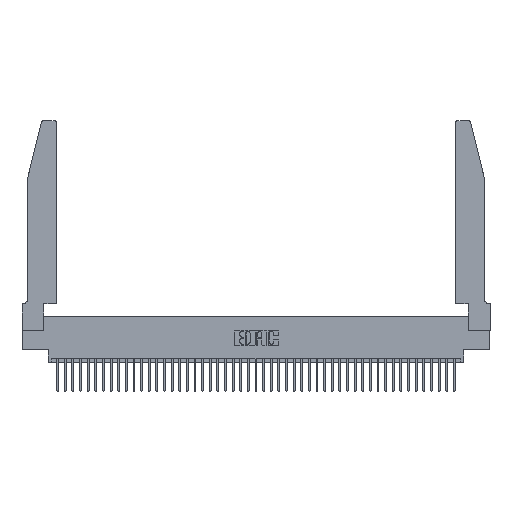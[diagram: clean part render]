
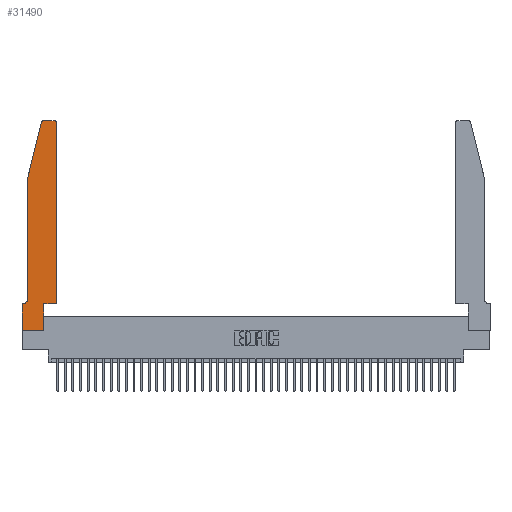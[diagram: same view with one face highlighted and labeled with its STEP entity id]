
A CAD part, top view. The second image highlights one B-rep face of the part: STEP entity #31490.
In plain terms, the highlighted planar face has unit normal (0, 0, 1).
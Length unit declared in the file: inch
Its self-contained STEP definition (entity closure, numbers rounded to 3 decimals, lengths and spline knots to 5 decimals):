
#122 = ORIENTED_EDGE ( 'NONE', *, *, #14981, .T. ) ;
#131 = AXIS2_PLACEMENT_3D ( 'NONE', #32396, #32083, #39551 ) ;
#266 = CARTESIAN_POINT ( 'NONE',  ( 0., 0., 0.37 ) ) ;
#344 = VERTEX_POINT ( 'NONE', #266 ) ;
#371 = VECTOR ( 'NONE', #37389, 39.37008 ) ;
#493 = LINE ( 'NONE', #6004, #3268 ) ;
#662 = CARTESIAN_POINT ( 'NONE',  ( 0.0755, 2., 0.37 ) ) ;
#692 = DIRECTION ( 'NONE',  ( 0., 1., 0. ) ) ;
#2466 = LINE ( 'NONE', #31133, #13912 ) ;
#3268 = VECTOR ( 'NONE', #34278, 39.37008 ) ;
#3992 = CARTESIAN_POINT ( 'NONE',  ( 0., 0.35, 0.37 ) ) ;
#4207 = VERTEX_POINT ( 'NONE', #3992 ) ;
#4444 = DIRECTION ( 'NONE',  ( 0., 0., 1. ) ) ;
#4799 = VERTEX_POINT ( 'NONE', #12134 ) ;
#5060 = CARTESIAN_POINT ( 'NONE',  ( 0.0755, 0.42, 0.37 ) ) ;
#5951 = CIRCLE ( 'NONE', #22077, 0.03 ) ;
#6004 = CARTESIAN_POINT ( 'NONE',  ( 0., 0., 0.37 ) ) ;
#6734 = DIRECTION ( 'NONE',  ( 0., -1., 0. ) ) ;
#6756 = CIRCLE ( 'NONE', #19233, 0.03 ) ;
#7800 = LINE ( 'NONE', #662, #24718 ) ;
#7810 = VERTEX_POINT ( 'NONE', #43664 ) ;
#9565 = CARTESIAN_POINT ( 'NONE',  ( 0.4205, 2.75, 0.37 ) ) ;
#10540 = ORIENTED_EDGE ( 'NONE', *, *, #13833, .T. ) ;
#11594 = CARTESIAN_POINT ( 'NONE',  ( 0., 0.35, 0.37 ) ) ;
#11911 = DIRECTION ( 'NONE',  ( 0., 1., 0. ) ) ;
#12134 = CARTESIAN_POINT ( 'NONE',  ( 0.0755, 2., 0.37 ) ) ;
#12741 = CARTESIAN_POINT ( 'NONE',  ( 0.284, 2.75, 0.37 ) ) ;
#12882 = DIRECTION ( 'NONE',  ( 1., 0., 0. ) ) ;
#13506 = LINE ( 'NONE', #35958, #35232 ) ;
#13753 = VERTEX_POINT ( 'NONE', #9565 ) ;
#13833 = EDGE_CURVE ( 'NONE', #28907, #7810, #15775, .T. ) ;
#13912 = VECTOR ( 'NONE', #44852, 39.37008 ) ;
#14045 = LINE ( 'NONE', #44385, #371 ) ;
#14304 = ORIENTED_EDGE ( 'NONE', *, *, #29888, .T. ) ;
#14630 = LINE ( 'NONE', #18368, #17883 ) ;
#14981 = EDGE_CURVE ( 'NONE', #4799, #15901, #13506, .T. ) ;
#15612 = EDGE_CURVE ( 'NONE', #15901, #42066, #16710, .T. ) ;
#15775 = LINE ( 'NONE', #36485, #27194 ) ;
#15901 = VERTEX_POINT ( 'NONE', #5060 ) ;
#16453 = ORIENTED_EDGE ( 'NONE', *, *, #36016, .T. ) ;
#16710 = CIRCLE ( 'NONE', #131, 0.07 ) ;
#16727 = VERTEX_POINT ( 'NONE', #12741 ) ;
#16975 = ORIENTED_EDGE ( 'NONE', *, *, #31848, .T. ) ;
#17883 = VECTOR ( 'NONE', #692, 39.37008 ) ;
#17894 = EDGE_LOOP ( 'NONE', ( #29249, #32715, #14304, #122, #44858, #43128, #21734, #16975, #24215, #10540, #25795, #16453 ) ) ;
#17975 = CARTESIAN_POINT ( 'NONE',  ( 0.4205, 2.72, 0.37 ) ) ;
#18368 = CARTESIAN_POINT ( 'NONE',  ( 0.2865, 0.35, 0.37 ) ) ;
#19233 = AXIS2_PLACEMENT_3D ( 'NONE', #17975, #42300, #38391 ) ;
#20474 = DIRECTION ( 'NONE',  ( -1., 0., 0. ) ) ;
#21734 = ORIENTED_EDGE ( 'NONE', *, *, #44191, .T. ) ;
#22077 = AXIS2_PLACEMENT_3D ( 'NONE', #43915, #23515, #12882 ) ;
#23265 = AXIS2_PLACEMENT_3D ( 'NONE', #11594, #4444, #28925 ) ;
#23515 = DIRECTION ( 'NONE',  ( 0., 0., 1. ) ) ;
#24188 = CARTESIAN_POINT ( 'NONE',  ( 0.2865, 0., 0.37 ) ) ;
#24215 = ORIENTED_EDGE ( 'NONE', *, *, #32094, .T. ) ;
#24718 = VECTOR ( 'NONE', #35835, 39.37008 ) ;
#25270 = PLANE ( 'NONE',  #23265 ) ;
#25594 = CARTESIAN_POINT ( 'NONE',  ( 0.4505, 0.35, 0.37 ) ) ;
#25795 = ORIENTED_EDGE ( 'NONE', *, *, #27388, .T. ) ;
#27194 = VECTOR ( 'NONE', #43634, 39.37008 ) ;
#27388 = EDGE_CURVE ( 'NONE', #7810, #41963, #29843, .T. ) ;
#27742 = VERTEX_POINT ( 'NONE', #24188 ) ;
#28102 = LINE ( 'NONE', #31256, #32437 ) ;
#28373 = FACE_OUTER_BOUND ( 'NONE', #17894, .T. ) ;
#28907 = VERTEX_POINT ( 'NONE', #37409 ) ;
#28925 = DIRECTION ( 'NONE',  ( 1., 0., 0. ) ) ;
#29245 = CARTESIAN_POINT ( 'NONE',  ( 0.25487, 2.72718, 0.37 ) ) ;
#29249 = ORIENTED_EDGE ( 'NONE', *, *, #30085, .T. ) ;
#29380 = CARTESIAN_POINT ( 'NONE',  ( 0.4505, 2.72, 0.37 ) ) ;
#29843 = LINE ( 'NONE', #25594, #41271 ) ;
#29888 = EDGE_CURVE ( 'NONE', #33630, #4799, #7800, .T. ) ;
#30085 = EDGE_CURVE ( 'NONE', #13753, #16727, #2466, .T. ) ;
#31133 = CARTESIAN_POINT ( 'NONE',  ( 0.2605, 2.75, 0.37 ) ) ;
#31256 = CARTESIAN_POINT ( 'NONE',  ( 0.0755, 0.35, 0.37 ) ) ;
#31490 = ADVANCED_FACE ( 'NONE', ( #28373 ), #25270, .T. ) ;
#31848 = EDGE_CURVE ( 'NONE', #344, #27742, #493, .T. ) ;
#32083 = DIRECTION ( 'NONE',  ( 0., 0., -1. ) ) ;
#32094 = EDGE_CURVE ( 'NONE', #27742, #28907, #14630, .T. ) ;
#32396 = CARTESIAN_POINT ( 'NONE',  ( 0.0055, 0.42, 0.37 ) ) ;
#32437 = VECTOR ( 'NONE', #20474, 39.37008 ) ;
#32715 = ORIENTED_EDGE ( 'NONE', *, *, #33256, .T. ) ;
#33256 = EDGE_CURVE ( 'NONE', #16727, #33630, #5951, .T. ) ;
#33630 = VERTEX_POINT ( 'NONE', #29245 ) ;
#33678 = CARTESIAN_POINT ( 'NONE',  ( 0.0055, 0.35, 0.37 ) ) ;
#34278 = DIRECTION ( 'NONE',  ( 1., 0., 0. ) ) ;
#35232 = VECTOR ( 'NONE', #6734, 39.37008 ) ;
#35835 = DIRECTION ( 'NONE',  ( -0.239, -0.971, 0. ) ) ;
#35958 = CARTESIAN_POINT ( 'NONE',  ( 0.0755, 2., 0.37 ) ) ;
#36016 = EDGE_CURVE ( 'NONE', #41963, #13753, #6756, .T. ) ;
#36485 = CARTESIAN_POINT ( 'NONE',  ( 0.4505, 0.35, 0.37 ) ) ;
#37389 = DIRECTION ( 'NONE',  ( 0., -1., 0. ) ) ;
#37409 = CARTESIAN_POINT ( 'NONE',  ( 0.2865, 0.35, 0.37 ) ) ;
#38391 = DIRECTION ( 'NONE',  ( 1., 0., 0. ) ) ;
#39551 = DIRECTION ( 'NONE',  ( -1., 0., 0. ) ) ;
#41271 = VECTOR ( 'NONE', #11911, 39.37008 ) ;
#41963 = VERTEX_POINT ( 'NONE', #29380 ) ;
#42066 = VERTEX_POINT ( 'NONE', #33678 ) ;
#42300 = DIRECTION ( 'NONE',  ( 0., 0., 1. ) ) ;
#43128 = ORIENTED_EDGE ( 'NONE', *, *, #44364, .T. ) ;
#43634 = DIRECTION ( 'NONE',  ( 1., 0., 0. ) ) ;
#43664 = CARTESIAN_POINT ( 'NONE',  ( 0.4505, 0.35, 0.37 ) ) ;
#43915 = CARTESIAN_POINT ( 'NONE',  ( 0.284, 2.72, 0.37 ) ) ;
#44191 = EDGE_CURVE ( 'NONE', #4207, #344, #14045, .T. ) ;
#44364 = EDGE_CURVE ( 'NONE', #42066, #4207, #28102, .T. ) ;
#44385 = CARTESIAN_POINT ( 'NONE',  ( 0., 0., 0.37 ) ) ;
#44852 = DIRECTION ( 'NONE',  ( -1., 0., 0. ) ) ;
#44858 = ORIENTED_EDGE ( 'NONE', *, *, #15612, .T. ) ;
